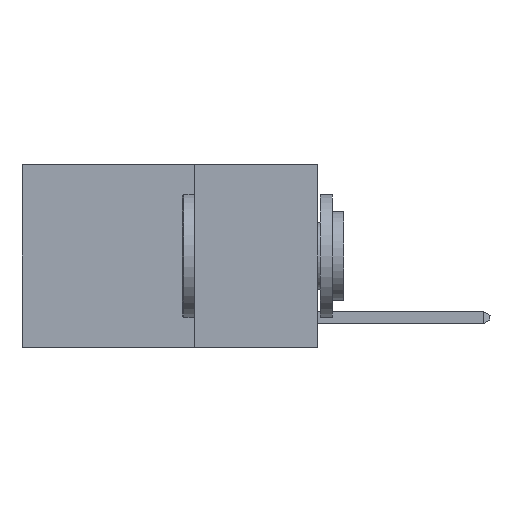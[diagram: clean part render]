
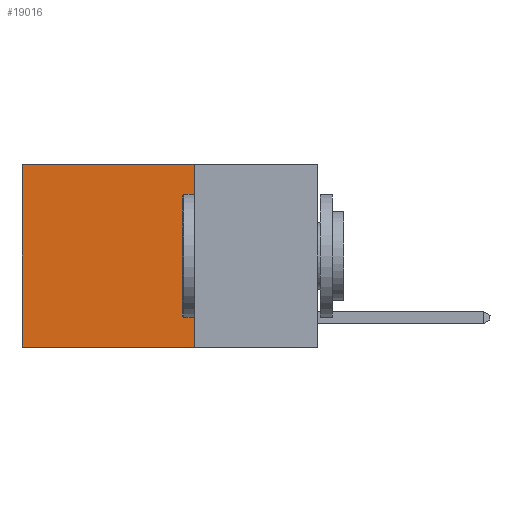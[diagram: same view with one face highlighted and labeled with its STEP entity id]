
A CAD part, left-side view. The second image highlights one B-rep face of the part: STEP entity #19016.
In plain terms, the highlighted planar face has unit normal (-1, 0, 0).
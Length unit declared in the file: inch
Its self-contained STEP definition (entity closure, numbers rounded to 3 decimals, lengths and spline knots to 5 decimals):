
#227 = FACE_OUTER_BOUND ( 'NONE', #18778, .T. ) ;
#2210 = CARTESIAN_POINT ( 'NONE',  ( 0.2625, 0.25, 0. ) ) ;
#2490 = LINE ( 'NONE', #17126, #14860 ) ;
#2851 = CARTESIAN_POINT ( 'NONE',  ( 0.2625, 0.25, 0. ) ) ;
#3093 = DIRECTION ( 'NONE',  ( 0., 1., 0. ) ) ;
#3208 = CARTESIAN_POINT ( 'NONE',  ( 0.2625, 0.6, 0. ) ) ;
#3570 = EDGE_CURVE ( 'NONE', #14689, #4032, #9574, .T. ) ;
#4032 = VERTEX_POINT ( 'NONE', #15379 ) ;
#4561 = VERTEX_POINT ( 'NONE', #17499 ) ;
#4759 = CARTESIAN_POINT ( 'NONE',  ( 0.2625, 0.25, -0.37 ) ) ;
#5036 = ORIENTED_EDGE ( 'NONE', *, *, #14398, .F. ) ;
#5310 = VECTOR ( 'NONE', #14534, 39.37008 ) ;
#5641 = VERTEX_POINT ( 'NONE', #9635 ) ;
#5854 = VECTOR ( 'NONE', #3093, 39.37008 ) ;
#5869 = DIRECTION ( 'NONE',  ( 0., 1., 0. ) ) ;
#8234 = EDGE_CURVE ( 'NONE', #5641, #4561, #16191, .T. ) ;
#8729 = DIRECTION ( 'NONE',  ( 0., 0., -1. ) ) ;
#8770 = DIRECTION ( 'NONE',  ( 0., 0., -1. ) ) ;
#9574 = LINE ( 'NONE', #2851, #19930 ) ;
#9635 = CARTESIAN_POINT ( 'NONE',  ( 0.2625, 0.25, -0.37 ) ) ;
#10213 = AXIS2_PLACEMENT_3D ( 'NONE', #2210, #15124, #8729 ) ;
#10488 = ORIENTED_EDGE ( 'NONE', *, *, #18551, .T. ) ;
#12342 = CARTESIAN_POINT ( 'NONE',  ( 0.2625, 0.25, 0. ) ) ;
#14075 = ORIENTED_EDGE ( 'NONE', *, *, #8234, .F. ) ;
#14398 = EDGE_CURVE ( 'NONE', #14689, #5641, #2490, .T. ) ;
#14534 = DIRECTION ( 'NONE',  ( 0., 0., -1. ) ) ;
#14689 = VERTEX_POINT ( 'NONE', #12342 ) ;
#14860 = VECTOR ( 'NONE', #8770, 39.37008 ) ;
#15124 = DIRECTION ( 'NONE',  ( 1., 0., 0. ) ) ;
#15379 = CARTESIAN_POINT ( 'NONE',  ( 0.2625, 0.6, 0. ) ) ;
#16191 = LINE ( 'NONE', #4759, #5854 ) ;
#17126 = CARTESIAN_POINT ( 'NONE',  ( 0.2625, 0.25, 0. ) ) ;
#17499 = CARTESIAN_POINT ( 'NONE',  ( 0.2625, 0.6, -0.37 ) ) ;
#18197 = LINE ( 'NONE', #3208, #5310 ) ;
#18551 = EDGE_CURVE ( 'NONE', #4032, #4561, #18197, .T. ) ;
#18778 = EDGE_LOOP ( 'NONE', ( #10488, #14075, #5036, #20485 ) ) ;
#19016 = ADVANCED_FACE ( 'NONE', ( #227 ), #19936, .F. ) ;
#19930 = VECTOR ( 'NONE', #5869, 39.37008 ) ;
#19936 = PLANE ( 'NONE',  #10213 ) ;
#20485 = ORIENTED_EDGE ( 'NONE', *, *, #3570, .T. ) ;
